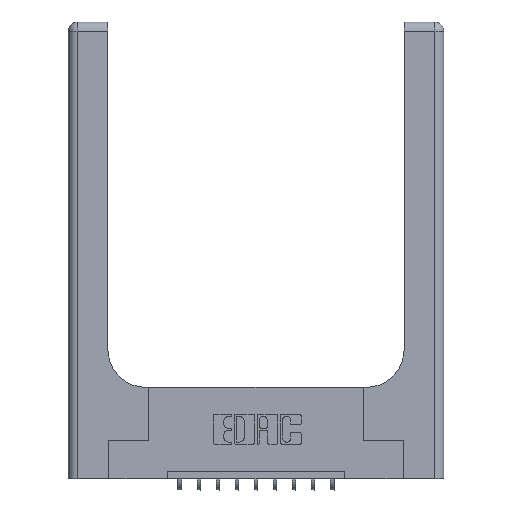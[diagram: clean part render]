
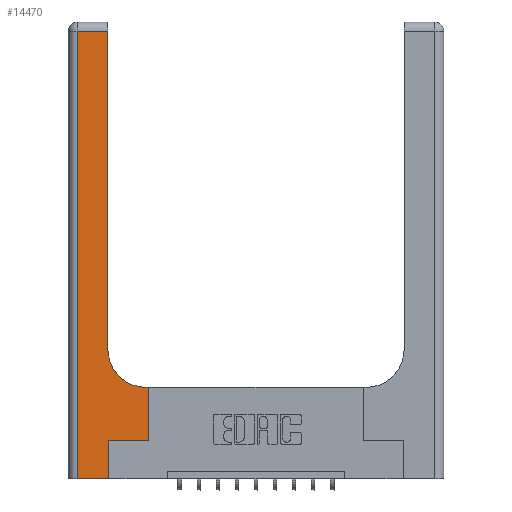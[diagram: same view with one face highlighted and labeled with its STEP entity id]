
A CAD part, top view. The second image highlights one B-rep face of the part: STEP entity #14470.
In plain terms, the highlighted planar face has unit normal (0, 0, 1).
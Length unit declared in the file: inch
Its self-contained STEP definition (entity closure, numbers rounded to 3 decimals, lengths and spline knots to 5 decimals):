
#92 = CARTESIAN_POINT ( 'NONE',  ( 0.06, 3., 0.37 ) ) ;
#183 = LINE ( 'NONE', #8541, #4043 ) ;
#274 = EDGE_CURVE ( 'NONE', #907, #14565, #7660, .T. ) ;
#391 = EDGE_LOOP ( 'NONE', ( #2694, #13815, #7496, #12007, #5588, #2909, #4444, #4430, #7673 ) ) ;
#532 = EDGE_CURVE ( 'NONE', #8657, #6478, #4525, .T. ) ;
#848 = LINE ( 'NONE', #15331, #1343 ) ;
#907 = VERTEX_POINT ( 'NONE', #14242 ) ;
#1012 = VECTOR ( 'NONE', #14912, 39.37008 ) ;
#1031 = VECTOR ( 'NONE', #14911, 39.37008 ) ;
#1167 = VECTOR ( 'NONE', #3408, 39.37008 ) ;
#1328 = EDGE_CURVE ( 'NONE', #2360, #4212, #848, .T. ) ;
#1343 = VECTOR ( 'NONE', #9426, 39.37008 ) ;
#1517 = CARTESIAN_POINT ( 'NONE',  ( 0., 3., 0.37 ) ) ;
#1602 = CARTESIAN_POINT ( 'NONE',  ( 0.26, 2.94, 0.37 ) ) ;
#1864 = VERTEX_POINT ( 'NONE', #1602 ) ;
#2360 = VERTEX_POINT ( 'NONE', #14475 ) ;
#2647 = CARTESIAN_POINT ( 'NONE',  ( 0.51, 0.85, 0.37 ) ) ;
#2662 = CARTESIAN_POINT ( 'NONE',  ( 0.265, 0.25, 0.37 ) ) ;
#2694 = ORIENTED_EDGE ( 'NONE', *, *, #8131, .T. ) ;
#2909 = ORIENTED_EDGE ( 'NONE', *, *, #15368, .T. ) ;
#3408 = DIRECTION ( 'NONE',  ( 0., 1., 0. ) ) ;
#3511 = VECTOR ( 'NONE', #8687, 39.37008 ) ;
#3891 = DIRECTION ( 'NONE',  ( 0., 0., -1. ) ) ;
#3914 = DIRECTION ( 'NONE',  ( 1., 0., 0. ) ) ;
#4043 = VECTOR ( 'NONE', #9662, 39.37008 ) ;
#4121 = CARTESIAN_POINT ( 'NONE',  ( 0.26, 0.85, 0.37 ) ) ;
#4204 = FACE_OUTER_BOUND ( 'NONE', #391, .T. ) ;
#4212 = VERTEX_POINT ( 'NONE', #4915 ) ;
#4301 = CARTESIAN_POINT ( 'NONE',  ( 0.265, 0., 0.37 ) ) ;
#4430 = ORIENTED_EDGE ( 'NONE', *, *, #1328, .T. ) ;
#4444 = ORIENTED_EDGE ( 'NONE', *, *, #12005, .T. ) ;
#4525 = LINE ( 'NONE', #8201, #15197 ) ;
#4915 = CARTESIAN_POINT ( 'NONE',  ( 0.51, 0.6, 0.37 ) ) ;
#4926 = CIRCLE ( 'NONE', #13866, 0.25 ) ;
#5199 = LINE ( 'NONE', #15146, #1031 ) ;
#5588 = ORIENTED_EDGE ( 'NONE', *, *, #532, .T. ) ;
#6183 = VERTEX_POINT ( 'NONE', #4121 ) ;
#6233 = DIRECTION ( 'NONE',  ( 0., 0., -1. ) ) ;
#6361 = VECTOR ( 'NONE', #7935, 39.37008 ) ;
#6478 = VERTEX_POINT ( 'NONE', #11038 ) ;
#7496 = ORIENTED_EDGE ( 'NONE', *, *, #274, .T. ) ;
#7599 = LINE ( 'NONE', #2662, #1012 ) ;
#7660 = LINE ( 'NONE', #92, #3511 ) ;
#7673 = ORIENTED_EDGE ( 'NONE', *, *, #10073, .T. ) ;
#7935 = DIRECTION ( 'NONE',  ( 1., 0., 0. ) ) ;
#8131 = EDGE_CURVE ( 'NONE', #6183, #1864, #183, .T. ) ;
#8190 = CARTESIAN_POINT ( 'NONE',  ( 0.528, 0.25, 0.37 ) ) ;
#8201 = CARTESIAN_POINT ( 'NONE',  ( 0.265, 0., 0.37 ) ) ;
#8541 = CARTESIAN_POINT ( 'NONE',  ( 0.26, 3., 0.37 ) ) ;
#8586 = CARTESIAN_POINT ( 'NONE',  ( 0.528, 0.25, 0.37 ) ) ;
#8657 = VERTEX_POINT ( 'NONE', #4301 ) ;
#8687 = DIRECTION ( 'NONE',  ( 0., -1., 0. ) ) ;
#8983 = PLANE ( 'NONE',  #12709 ) ;
#9101 = EDGE_CURVE ( 'NONE', #1864, #907, #5199, .T. ) ;
#9197 = CARTESIAN_POINT ( 'NONE',  ( 0., 0., 0.37 ) ) ;
#9371 = LINE ( 'NONE', #8190, #1167 ) ;
#9426 = DIRECTION ( 'NONE',  ( -1., 0., 0. ) ) ;
#9662 = DIRECTION ( 'NONE',  ( 0., 1., 0. ) ) ;
#10073 = EDGE_CURVE ( 'NONE', #4212, #6183, #4926, .T. ) ;
#10285 = DIRECTION ( 'NONE',  ( -1., 0., 0. ) ) ;
#10557 = VERTEX_POINT ( 'NONE', #8586 ) ;
#11038 = CARTESIAN_POINT ( 'NONE',  ( 0.265, 0.25, 0.37 ) ) ;
#12005 = EDGE_CURVE ( 'NONE', #10557, #2360, #9371, .T. ) ;
#12007 = ORIENTED_EDGE ( 'NONE', *, *, #13927, .T. ) ;
#12709 = AXIS2_PLACEMENT_3D ( 'NONE', #1517, #3891, #10285 ) ;
#13705 = CARTESIAN_POINT ( 'NONE',  ( 0.06, 0., 0.37 ) ) ;
#13815 = ORIENTED_EDGE ( 'NONE', *, *, #9101, .T. ) ;
#13866 = AXIS2_PLACEMENT_3D ( 'NONE', #2647, #6233, #3914 ) ;
#13927 = EDGE_CURVE ( 'NONE', #14565, #8657, #15252, .T. ) ;
#14242 = CARTESIAN_POINT ( 'NONE',  ( 0.06, 2.94, 0.37 ) ) ;
#14470 = ADVANCED_FACE ( 'NONE', ( #4204 ), #8983, .F. ) ;
#14475 = CARTESIAN_POINT ( 'NONE',  ( 0.528, 0.6, 0.37 ) ) ;
#14565 = VERTEX_POINT ( 'NONE', #13705 ) ;
#14911 = DIRECTION ( 'NONE',  ( -1., 0., 0. ) ) ;
#14912 = DIRECTION ( 'NONE',  ( 1., 0., 0. ) ) ;
#15146 = CARTESIAN_POINT ( 'NONE',  ( 0., 2.94, 0.37 ) ) ;
#15197 = VECTOR ( 'NONE', #15600, 39.37008 ) ;
#15252 = LINE ( 'NONE', #9197, #6361 ) ;
#15331 = CARTESIAN_POINT ( 'NONE',  ( 0.26, 0.6, 0.37 ) ) ;
#15368 = EDGE_CURVE ( 'NONE', #6478, #10557, #7599, .T. ) ;
#15600 = DIRECTION ( 'NONE',  ( 0., 1., 0. ) ) ;
